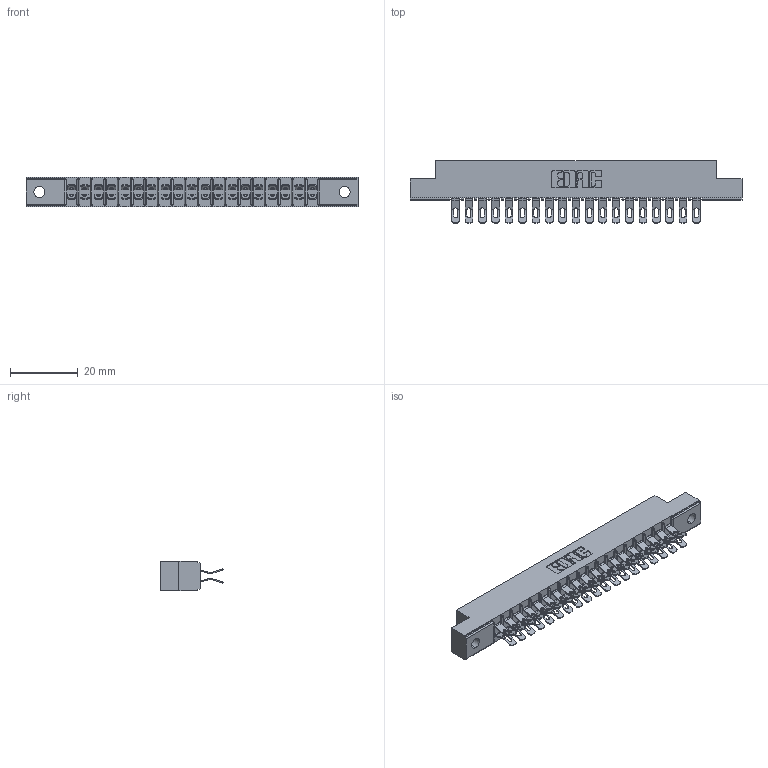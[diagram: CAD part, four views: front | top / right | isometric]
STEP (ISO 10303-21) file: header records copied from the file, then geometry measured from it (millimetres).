
FILE_DESCRIPTION (( 'STEP AP203' ), '1' );
FILE_NAME ('315-038-555-202.STEP', '2019-09-10T17:08:01', ( '' ), ( '' ), 'SwSTEP 2.0', 'SolidWorks 2016', '' );
FILE_SCHEMA (( 'CONFIG_CONTROL_DESIGN' ));
Length unit declared in the file: inch
Products named in the file (3): 315-038-555-202; 305-290-001_555; 305 Part_.128 Dia
Assembly tree (39 placements, depth 2):
  315-038-555-202
    305 Part_.128 Dia
    305-290-001_555  x38
Bounding box: 98.3 x 18.41 x 8.71 mm (x, y, z)
Volume: 6249 mm3; surface area: 12006.2 mm2
Topology: 39 solids, 39 shells, 2624 faces, 7821 edges, 5110 vertices
Faces by surface type: plane 1284, cylinder 1264, sphere 76
Entity records: 23998 total; most frequent: CARTESIAN_POINT 3989, ORIENTED_EDGE 3946, DIRECTION 3871, EDGE_CURVE 1973, VECTOR 1551, LINE 1551, VERTEX_POINT 1262, AXIS2_PLACEMENT_3D 1160
